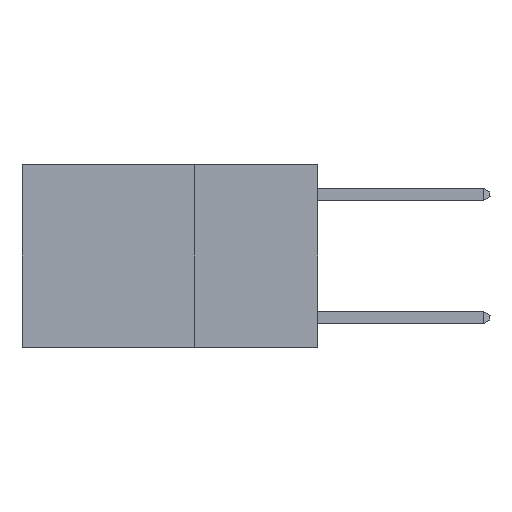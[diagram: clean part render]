
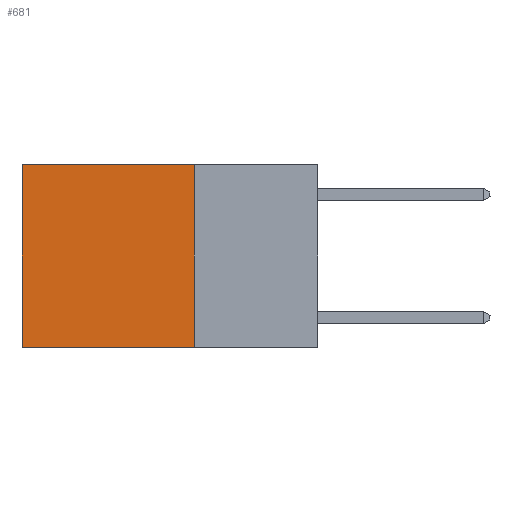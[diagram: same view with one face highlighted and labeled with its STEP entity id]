
A CAD part, left-side view. The second image highlights one B-rep face of the part: STEP entity #681.
In plain terms, the highlighted planar face has unit normal (-1, 0, 0).
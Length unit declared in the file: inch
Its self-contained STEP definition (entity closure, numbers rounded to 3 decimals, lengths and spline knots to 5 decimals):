
#315 = CARTESIAN_POINT ( 'NONE',  ( 0.2625, 0.25, 0. ) ) ;
#500 = EDGE_CURVE ( 'NONE', #14270, #14238, #12247, .T. ) ;
#681 = ADVANCED_FACE ( 'NONE', ( #10410 ), #3794, .F. ) ;
#1697 = CARTESIAN_POINT ( 'NONE',  ( 0.2625, 0.25, 0. ) ) ;
#2880 = CARTESIAN_POINT ( 'NONE',  ( 0.2625, 0.25, -0.37 ) ) ;
#3625 = CARTESIAN_POINT ( 'NONE',  ( 0.2625, 0.6, 0. ) ) ;
#3638 = VECTOR ( 'NONE', #4019, 39.37008 ) ;
#3707 = CARTESIAN_POINT ( 'NONE',  ( 0.2625, 0.25, 0. ) ) ;
#3794 = PLANE ( 'NONE',  #11424 ) ;
#4019 = DIRECTION ( 'NONE',  ( 0., 1., 0. ) ) ;
#4267 = LINE ( 'NONE', #1697, #3638 ) ;
#5098 = CARTESIAN_POINT ( 'NONE',  ( 0.2625, 0.6, -0.37 ) ) ;
#5151 = DIRECTION ( 'NONE',  ( 1., 0., 0. ) ) ;
#5215 = CARTESIAN_POINT ( 'NONE',  ( 0.2625, 0.25, -0.37 ) ) ;
#7057 = LINE ( 'NONE', #9800, #15630 ) ;
#7234 = VERTEX_POINT ( 'NONE', #3707 ) ;
#7338 = ORIENTED_EDGE ( 'NONE', *, *, #12953, .F. ) ;
#7426 = DIRECTION ( 'NONE',  ( 0., 0., -1. ) ) ;
#7854 = DIRECTION ( 'NONE',  ( 0., 0., -1. ) ) ;
#8098 = LINE ( 'NONE', #2880, #9178 ) ;
#8761 = EDGE_CURVE ( 'NONE', #12661, #14238, #8098, .T. ) ;
#8920 = ORIENTED_EDGE ( 'NONE', *, *, #8761, .F. ) ;
#9178 = VECTOR ( 'NONE', #14493, 39.37008 ) ;
#9800 = CARTESIAN_POINT ( 'NONE',  ( 0.2625, 0.25, 0. ) ) ;
#10410 = FACE_OUTER_BOUND ( 'NONE', #14526, .T. ) ;
#11424 = AXIS2_PLACEMENT_3D ( 'NONE', #315, #5151, #7854 ) ;
#11635 = EDGE_CURVE ( 'NONE', #7234, #14270, #4267, .T. ) ;
#11958 = VECTOR ( 'NONE', #7426, 39.37008 ) ;
#12247 = LINE ( 'NONE', #3625, #11958 ) ;
#12297 = DIRECTION ( 'NONE',  ( 0., 0., -1. ) ) ;
#12661 = VERTEX_POINT ( 'NONE', #5215 ) ;
#12699 = ORIENTED_EDGE ( 'NONE', *, *, #11635, .T. ) ;
#12707 = CARTESIAN_POINT ( 'NONE',  ( 0.2625, 0.6, 0. ) ) ;
#12824 = ORIENTED_EDGE ( 'NONE', *, *, #500, .T. ) ;
#12953 = EDGE_CURVE ( 'NONE', #7234, #12661, #7057, .T. ) ;
#14238 = VERTEX_POINT ( 'NONE', #5098 ) ;
#14270 = VERTEX_POINT ( 'NONE', #12707 ) ;
#14493 = DIRECTION ( 'NONE',  ( 0., 1., 0. ) ) ;
#14526 = EDGE_LOOP ( 'NONE', ( #12824, #8920, #7338, #12699 ) ) ;
#15630 = VECTOR ( 'NONE', #12297, 39.37008 ) ;
